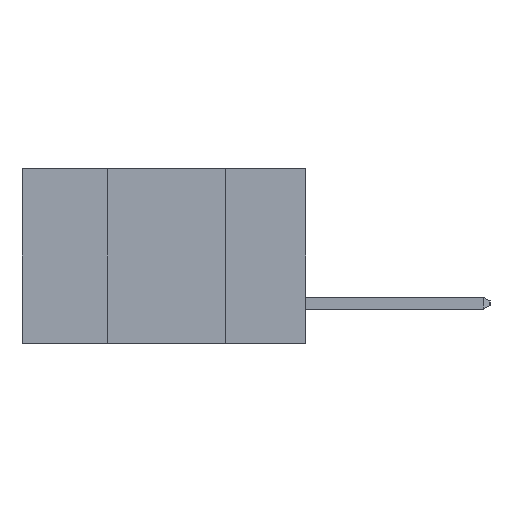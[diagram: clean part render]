
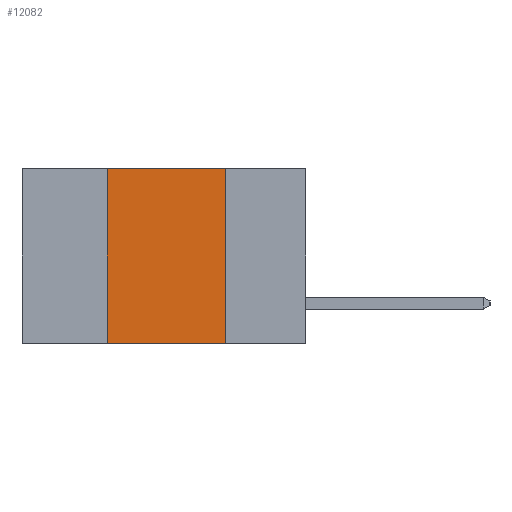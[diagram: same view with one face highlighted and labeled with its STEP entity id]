
A CAD part, left-side view. The second image highlights one B-rep face of the part: STEP entity #12082.
In plain terms, the highlighted planar face has unit normal (-1, 0, 0).
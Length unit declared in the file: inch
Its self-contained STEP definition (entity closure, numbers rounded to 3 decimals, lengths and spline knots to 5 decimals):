
#445 = DIRECTION ( 'NONE',  ( 0., 0., -1. ) ) ;
#1452 = DIRECTION ( 'NONE',  ( 0., -1., 0. ) ) ;
#2827 = EDGE_CURVE ( 'NONE', #14538, #8368, #7045, .T. ) ;
#3110 = DIRECTION ( 'NONE',  ( 0., -1., 0. ) ) ;
#3480 = CARTESIAN_POINT ( 'NONE',  ( 0., 0.6, 0. ) ) ;
#4066 = CARTESIAN_POINT ( 'NONE',  ( 0., 0.17, -0.37 ) ) ;
#4225 = CARTESIAN_POINT ( 'NONE',  ( 0., 0.17, 0. ) ) ;
#4381 = CARTESIAN_POINT ( 'NONE',  ( 0., 0.42, -0.37 ) ) ;
#4805 = AXIS2_PLACEMENT_3D ( 'NONE', #6708, #7909, #445 ) ;
#5817 = VERTEX_POINT ( 'NONE', #4381 ) ;
#5963 = VECTOR ( 'NONE', #1452, 39.37008 ) ;
#6591 = LINE ( 'NONE', #4066, #12590 ) ;
#6708 = CARTESIAN_POINT ( 'NONE',  ( 0., 0.6, 0. ) ) ;
#7045 = LINE ( 'NONE', #3480, #13033 ) ;
#7136 = DIRECTION ( 'NONE',  ( 0., 0., 1. ) ) ;
#7584 = EDGE_CURVE ( 'NONE', #5817, #12329, #9166, .T. ) ;
#7909 = DIRECTION ( 'NONE',  ( 1., 0., 0. ) ) ;
#8368 = VERTEX_POINT ( 'NONE', #4225 ) ;
#8881 = VECTOR ( 'NONE', #7136, 39.37008 ) ;
#9157 = FACE_OUTER_BOUND ( 'NONE', #14602, .T. ) ;
#9166 = LINE ( 'NONE', #11319, #5963 ) ;
#10161 = DIRECTION ( 'NONE',  ( 0., 0., -1. ) ) ;
#10217 = EDGE_CURVE ( 'NONE', #8368, #12329, #6591, .T. ) ;
#11319 = CARTESIAN_POINT ( 'NONE',  ( 0., 0.6, -0.37 ) ) ;
#11736 = LINE ( 'NONE', #14262, #8881 ) ;
#12082 = ADVANCED_FACE ( 'NONE', ( #9157 ), #14996, .F. ) ;
#12329 = VERTEX_POINT ( 'NONE', #14290 ) ;
#12590 = VECTOR ( 'NONE', #10161, 39.37008 ) ;
#13033 = VECTOR ( 'NONE', #3110, 39.37008 ) ;
#13242 = ORIENTED_EDGE ( 'NONE', *, *, #2827, .F. ) ;
#14262 = CARTESIAN_POINT ( 'NONE',  ( 0., 0.42, -0.37 ) ) ;
#14290 = CARTESIAN_POINT ( 'NONE',  ( 0., 0.17, -0.37 ) ) ;
#14446 = EDGE_CURVE ( 'NONE', #5817, #14538, #11736, .T. ) ;
#14538 = VERTEX_POINT ( 'NONE', #15552 ) ;
#14602 = EDGE_LOOP ( 'NONE', ( #15444, #13242, #15510, #15166 ) ) ;
#14996 = PLANE ( 'NONE',  #4805 ) ;
#15166 = ORIENTED_EDGE ( 'NONE', *, *, #7584, .T. ) ;
#15444 = ORIENTED_EDGE ( 'NONE', *, *, #10217, .F. ) ;
#15510 = ORIENTED_EDGE ( 'NONE', *, *, #14446, .F. ) ;
#15552 = CARTESIAN_POINT ( 'NONE',  ( 0., 0.42, 0. ) ) ;
